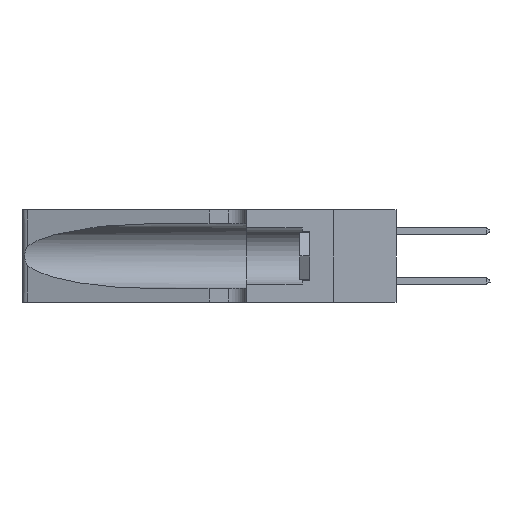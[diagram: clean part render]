
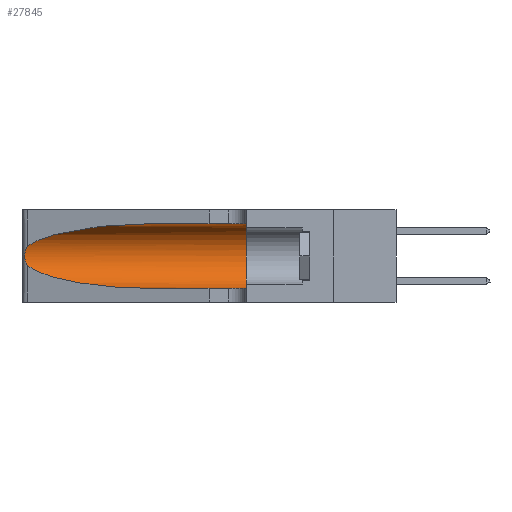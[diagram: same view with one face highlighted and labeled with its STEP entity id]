
A CAD part, left-side view. The second image highlights one B-rep face of the part: STEP entity #27845.
In plain terms, the highlighted cylindrical face has radius 3.308 mm (diameter 6.617 mm), a partial arc.
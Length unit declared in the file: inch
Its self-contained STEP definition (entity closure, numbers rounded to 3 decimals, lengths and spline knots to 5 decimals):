
#343 = VERTEX_POINT ( 'NONE', #2584 ) ;
#757 = CARTESIAN_POINT ( 'NONE',  ( 0.1305, 0.72297, 0.31525 ) ) ;
#1554 = DIRECTION ( 'NONE',  ( 0., 0., -1. ) ) ;
#1929 = CARTESIAN_POINT ( 'NONE',  ( 0.25487, 1.22718, 0.22369 ) ) ;
#2274 = CARTESIAN_POINT ( 'NONE',  ( 0.25787, 1.23484, 0.2124 ) ) ;
#2584 = CARTESIAN_POINT ( 'NONE',  ( 0.1305, 0.35, 0.05475 ) ) ;
#3077 = VERTEX_POINT ( 'NONE', #8546 ) ;
#4423 = VERTEX_POINT ( 'NONE', #32544 ) ;
#4435 = ORIENTED_EDGE ( 'NONE', *, *, #27296, .T. ) ;
#4474 = ORIENTED_EDGE ( 'NONE', *, *, #27274, .T. ) ;
#4652 = EDGE_CURVE ( 'NONE', #36031, #343, #35457, .T. ) ;
#4754 = DIRECTION ( 'NONE',  ( 0., -1., 0. ) ) ;
#5301 = CARTESIAN_POINT ( 'NONE',  ( 0.26018, 1.23835, 0.19895 ) ) ;
#6609 =( BOUNDED_CURVE ( )  B_SPLINE_CURVE ( 3, ( #11008, #28831, #31769, #13998 ),
 .UNSPECIFIED., .F., .F. ) 
 B_SPLINE_CURVE_WITH_KNOTS ( ( 4, 4 ),
 ( 3.44316, 4.71239 ),
 .UNSPECIFIED. ) 
 CURVE ( )  GEOMETRIC_REPRESENTATION_ITEM ( )  RATIONAL_B_SPLINE_CURVE ( ( 1., 0.87, 0.87, 1. ) ) 
 REPRESENTATION_ITEM ( '' )  );
#6638 = EDGE_CURVE ( 'NONE', #4423, #343, #18255, .T. ) ;
#7861 = VECTOR ( 'NONE', #38309, 39.37008 ) ;
#8240 = CARTESIAN_POINT ( 'NONE',  ( 0.26075, 1.23896, 0.178 ) ) ;
#8546 = CARTESIAN_POINT ( 'NONE',  ( 0.25487, 1.22718, 0.14631 ) ) ;
#8785 = LINE ( 'NONE', #14711, #7861 ) ;
#9835 = DIRECTION ( 'NONE',  ( 0., 1., 0. ) ) ;
#10283 = VECTOR ( 'NONE', #10478, 39.37008 ) ;
#10463 = CARTESIAN_POINT ( 'NONE',  ( 0.1305, 0.35, 0.31525 ) ) ;
#10478 = DIRECTION ( 'NONE',  ( 0., -1., 0. ) ) ;
#11008 = CARTESIAN_POINT ( 'NONE',  ( 0.25487, 1.22718, 0.14631 ) ) ;
#11079 = ORIENTED_EDGE ( 'NONE', *, *, #20688, .F. ) ;
#11263 = CARTESIAN_POINT ( 'NONE',  ( 0.25856, 1.23593, 0.16098 ) ) ;
#13112 = VERTEX_POINT ( 'NONE', #28447 ) ;
#13998 = CARTESIAN_POINT ( 'NONE',  ( 0.1305, 0.72297, 0.05475 ) ) ;
#14127 = CARTESIAN_POINT ( 'NONE',  ( 0.25555, 1.22994, 0.2215 ) ) ;
#14257 = CARTESIAN_POINT ( 'NONE',  ( 0.25639, 1.23186, 0.15144 ) ) ;
#14711 = CARTESIAN_POINT ( 'NONE',  ( 0.1305, 1.61858, 0.31525 ) ) ;
#15280 = CYLINDRICAL_SURFACE ( 'NONE', #35114, 0.13025 ) ;
#15793 = CARTESIAN_POINT ( 'NONE',  ( 0.2373, 1.15595, 0.28018 ) ) ;
#16225 = FACE_OUTER_BOUND ( 'NONE', #23167, .T. ) ;
#16559 = CARTESIAN_POINT ( 'NONE',  ( 0.1305, 1.61858, 0.185 ) ) ;
#17264 = CARTESIAN_POINT ( 'NONE',  ( 0.25487, 1.22718, 0.14631 ) ) ;
#18255 = LINE ( 'NONE', #22338, #10283 ) ;
#19508 = AXIS2_PLACEMENT_3D ( 'NONE', #27683, #9835, #30613 ) ;
#20139 = CARTESIAN_POINT ( 'NONE',  ( 0.25639, 1.23184, 0.21858 ) ) ;
#20688 = EDGE_CURVE ( 'NONE', #13112, #36031, #8785, .T. ) ;
#21000 = ORIENTED_EDGE ( 'NONE', *, *, #36589, .T. ) ;
#22338 = CARTESIAN_POINT ( 'NONE',  ( 0.1305, 1.61858, 0.05475 ) ) ;
#23117 = CARTESIAN_POINT ( 'NONE',  ( 0.25854, 1.2359, 0.20912 ) ) ;
#23167 = EDGE_LOOP ( 'NONE', ( #21000, #4435, #4474, #36257, #36996, #11079 ) ) ;
#24659 = CARTESIAN_POINT ( 'NONE',  ( 0.18966, 0.96281, 0.31525 ) ) ;
#26091 = CARTESIAN_POINT ( 'NONE',  ( 0.26075, 1.23896, 0.19203 ) ) ;
#26634 = VERTEX_POINT ( 'NONE', #1929 ) ;
#27274 = EDGE_CURVE ( 'NONE', #3077, #4423, #6609, .T. ) ;
#27296 = EDGE_CURVE ( 'NONE', #26634, #3077, #29045, .T. ) ;
#27683 = CARTESIAN_POINT ( 'NONE',  ( 0.1305, 0.35, 0.185 ) ) ;
#27845 = ADVANCED_FACE ( 'NONE', ( #16225 ), #15280, .F. ) ;
#28447 = CARTESIAN_POINT ( 'NONE',  ( 0.1305, 0.72297, 0.31525 ) ) ;
#28831 = CARTESIAN_POINT ( 'NONE',  ( 0.2373, 1.15595, 0.08982 ) ) ;
#29045 = B_SPLINE_CURVE_WITH_KNOTS ( 'NONE', 3,
 ( #34814, #14127, #20139, #2274, #23117, #5301, #26091, #8240, #29077, #11263, #32018, #14257, #34935, #17264 ),
 .UNSPECIFIED., .F., .F.,
 ( 4, 2, 2, 2, 2, 2, 4 ),
 ( 0., 0.00027, 0.00053, 0.00107, 0.0016, 0.00187, 0.00214 ),
 .UNSPECIFIED. ) ;
#29077 = CARTESIAN_POINT ( 'NONE',  ( 0.26017, 1.23833, 0.17102 ) ) ;
#30613 = DIRECTION ( 'NONE',  ( 0., 0., 1. ) ) ;
#31235 =( BOUNDED_CURVE ( )  B_SPLINE_CURVE ( 3, ( #757, #24659, #15793, #36423 ),
 .UNSPECIFIED., .F., .F. ) 
 B_SPLINE_CURVE_WITH_KNOTS ( ( 4, 4 ),
 ( 1.5708, 2.84003 ),
 .UNSPECIFIED. ) 
 CURVE ( )  GEOMETRIC_REPRESENTATION_ITEM ( )  RATIONAL_B_SPLINE_CURVE ( ( 1., 0.87, 0.87, 1. ) ) 
 REPRESENTATION_ITEM ( '' )  );
#31769 = CARTESIAN_POINT ( 'NONE',  ( 0.18966, 0.96281, 0.05475 ) ) ;
#32018 = CARTESIAN_POINT ( 'NONE',  ( 0.25789, 1.23486, 0.15765 ) ) ;
#32544 = CARTESIAN_POINT ( 'NONE',  ( 0.1305, 0.72297, 0.05475 ) ) ;
#34814 = CARTESIAN_POINT ( 'NONE',  ( 0.25487, 1.22718, 0.22369 ) ) ;
#34935 = CARTESIAN_POINT ( 'NONE',  ( 0.25555, 1.22993, 0.14849 ) ) ;
#35114 = AXIS2_PLACEMENT_3D ( 'NONE', #16559, #4754, #1554 ) ;
#35457 = CIRCLE ( 'NONE', #19508, 0.13025 ) ;
#36031 = VERTEX_POINT ( 'NONE', #10463 ) ;
#36257 = ORIENTED_EDGE ( 'NONE', *, *, #6638, .T. ) ;
#36423 = CARTESIAN_POINT ( 'NONE',  ( 0.25487, 1.22718, 0.22369 ) ) ;
#36589 = EDGE_CURVE ( 'NONE', #13112, #26634, #31235, .T. ) ;
#36996 = ORIENTED_EDGE ( 'NONE', *, *, #4652, .F. ) ;
#38309 = DIRECTION ( 'NONE',  ( 0., -1., 0. ) ) ;
